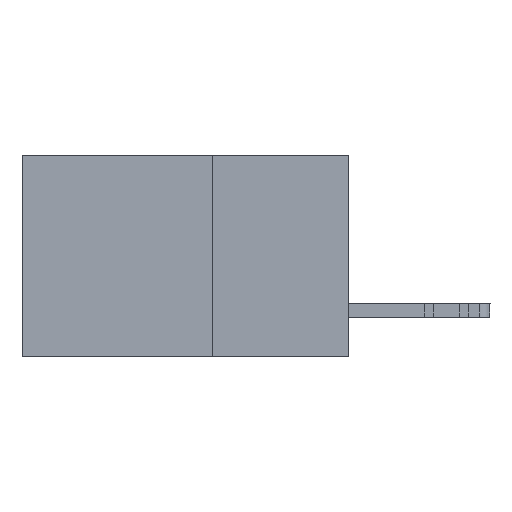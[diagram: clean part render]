
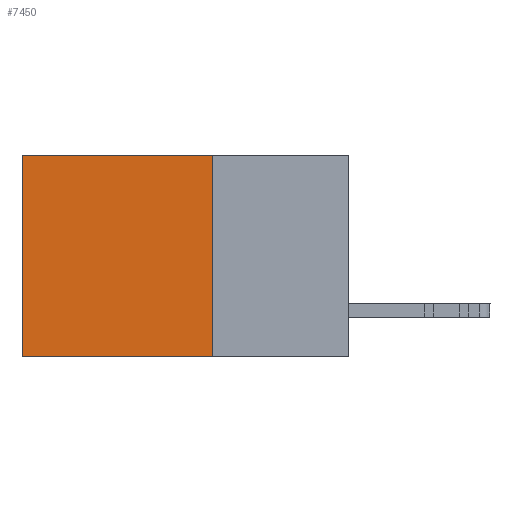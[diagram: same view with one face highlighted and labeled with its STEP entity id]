
A CAD part, left-side view. The second image highlights one B-rep face of the part: STEP entity #7450.
In plain terms, the highlighted planar face has unit normal (-1, 0, 0).
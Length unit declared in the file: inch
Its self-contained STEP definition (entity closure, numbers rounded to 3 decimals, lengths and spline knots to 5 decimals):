
#631 = VERTEX_POINT ( 'NONE', #17332 ) ;
#693 = ORIENTED_EDGE ( 'NONE', *, *, #9830, .T. ) ;
#1420 = DIRECTION ( 'NONE',  ( 0., 0., -1. ) ) ;
#1748 = DIRECTION ( 'NONE',  ( 0., 0., -1. ) ) ;
#1875 = FACE_OUTER_BOUND ( 'NONE', #6116, .T. ) ;
#2440 = LINE ( 'NONE', #2568, #8202 ) ;
#2568 = CARTESIAN_POINT ( 'NONE',  ( 0.2615, 0.6, -0.37 ) ) ;
#3731 = DIRECTION ( 'NONE',  ( 0., 1., 0. ) ) ;
#5132 = ORIENTED_EDGE ( 'NONE', *, *, #19424, .T. ) ;
#5181 = PLANE ( 'NONE',  #18191 ) ;
#6116 = EDGE_LOOP ( 'NONE', ( #5132, #8860, #12948, #693 ) ) ;
#6201 = DIRECTION ( 'NONE',  ( 0., 0., -1. ) ) ;
#6252 = LINE ( 'NONE', #13425, #22493 ) ;
#6907 = VERTEX_POINT ( 'NONE', #12107 ) ;
#7450 = ADVANCED_FACE ( 'NONE', ( #1875 ), #5181, .F. ) ;
#8202 = VECTOR ( 'NONE', #6201, 39.37008 ) ;
#8860 = ORIENTED_EDGE ( 'NONE', *, *, #19849, .F. ) ;
#9830 = EDGE_CURVE ( 'NONE', #631, #6907, #16324, .T. ) ;
#10343 = CARTESIAN_POINT ( 'NONE',  ( 0.2615, 0.25, -0.37 ) ) ;
#11034 = CARTESIAN_POINT ( 'NONE',  ( 0.2615, 0.25, 0. ) ) ;
#12107 = CARTESIAN_POINT ( 'NONE',  ( 0.2615, 0.6, 0. ) ) ;
#12948 = ORIENTED_EDGE ( 'NONE', *, *, #20715, .F. ) ;
#13106 = VECTOR ( 'NONE', #1420, 39.37008 ) ;
#13425 = CARTESIAN_POINT ( 'NONE',  ( 0.2615, 0.25, -0.37 ) ) ;
#13810 = CARTESIAN_POINT ( 'NONE',  ( 0.2615, 0.6, -0.37 ) ) ;
#16324 = LINE ( 'NONE', #11034, #16366 ) ;
#16366 = VECTOR ( 'NONE', #3731, 39.37008 ) ;
#17332 = CARTESIAN_POINT ( 'NONE',  ( 0.2615, 0.25, 0. ) ) ;
#18191 = AXIS2_PLACEMENT_3D ( 'NONE', #23063, #21503, #1748 ) ;
#18761 = VERTEX_POINT ( 'NONE', #19574 ) ;
#19424 = EDGE_CURVE ( 'NONE', #6907, #21929, #2440, .T. ) ;
#19574 = CARTESIAN_POINT ( 'NONE',  ( 0.2615, 0.25, -0.37 ) ) ;
#19849 = EDGE_CURVE ( 'NONE', #18761, #21929, #6252, .T. ) ;
#20615 = DIRECTION ( 'NONE',  ( 0., 1., 0. ) ) ;
#20715 = EDGE_CURVE ( 'NONE', #631, #18761, #20855, .T. ) ;
#20855 = LINE ( 'NONE', #10343, #13106 ) ;
#21503 = DIRECTION ( 'NONE',  ( 1., 0., 0. ) ) ;
#21929 = VERTEX_POINT ( 'NONE', #13810 ) ;
#22493 = VECTOR ( 'NONE', #20615, 39.37008 ) ;
#23063 = CARTESIAN_POINT ( 'NONE',  ( 0.2615, 0.25, -0.37 ) ) ;
